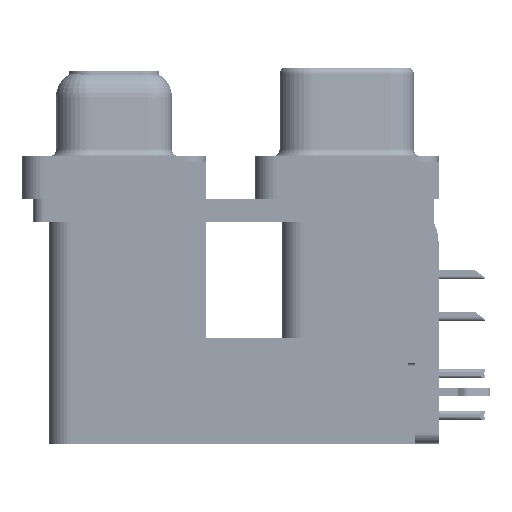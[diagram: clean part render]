
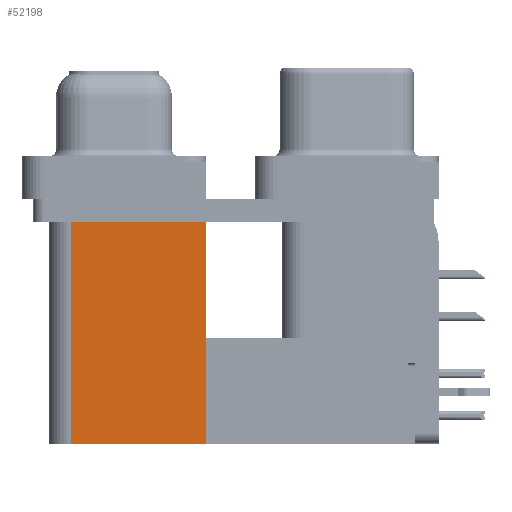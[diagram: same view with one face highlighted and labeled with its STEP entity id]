
A CAD part, left-side view. The second image highlights one B-rep face of the part: STEP entity #52198.
In plain terms, the highlighted planar face has unit normal (-1, 0, 0).
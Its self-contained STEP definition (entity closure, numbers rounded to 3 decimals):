
#2937 = CARTESIAN_POINT ( 'NONE',  ( 3.79, 18.8, -19.2 ) ) ;
#3347 = EDGE_LOOP ( 'NONE', ( #26915, #19031, #13800, #28448 ) ) ;
#3531 = EDGE_CURVE ( 'NONE', #57942, #61776, #18098, .T. ) ;
#4173 = CARTESIAN_POINT ( 'NONE',  ( 3.79, 9.6, -19.2 ) ) ;
#6087 = AXIS2_PLACEMENT_3D ( 'NONE', #23363, #63778, #54277 ) ;
#10407 = EDGE_CURVE ( 'NONE', #13706, #61776, #45657, .T. ) ;
#13706 = VERTEX_POINT ( 'NONE', #2937 ) ;
#13800 = ORIENTED_EDGE ( 'NONE', *, *, #35680, .F. ) ;
#14604 = CARTESIAN_POINT ( 'NONE',  ( 3.79, 18.8, -2.5 ) ) ;
#18098 = LINE ( 'NONE', #38801, #58396 ) ;
#19031 = ORIENTED_EDGE ( 'NONE', *, *, #10407, .F. ) ;
#21102 = CARTESIAN_POINT ( 'NONE',  ( 3.79, 9.6, -19.2 ) ) ;
#23363 = CARTESIAN_POINT ( 'NONE',  ( 3.79, 9.6, -19.2 ) ) ;
#26915 = ORIENTED_EDGE ( 'NONE', *, *, #3531, .T. ) ;
#27692 = EDGE_CURVE ( 'NONE', #57600, #57942, #54290, .T. ) ;
#28448 = ORIENTED_EDGE ( 'NONE', *, *, #27692, .T. ) ;
#29722 = CARTESIAN_POINT ( 'NONE',  ( 3.79, 18.8, -19.2 ) ) ;
#32843 = VECTOR ( 'NONE', #50386, 1000. ) ;
#35680 = EDGE_CURVE ( 'NONE', #57600, #13706, #51727, .T. ) ;
#38801 = CARTESIAN_POINT ( 'NONE',  ( 3.79, 9.6, -2.5 ) ) ;
#39457 = VECTOR ( 'NONE', #44085, 1000. ) ;
#43736 = PLANE ( 'NONE',  #6087 ) ;
#44085 = DIRECTION ( 'NONE',  ( 0., 0., 1. ) ) ;
#45657 = LINE ( 'NONE', #29722, #58118 ) ;
#49173 = CARTESIAN_POINT ( 'NONE',  ( 3.79, 9.6, -19.2 ) ) ;
#50386 = DIRECTION ( 'NONE',  ( 0., 1., 0. ) ) ;
#50420 = DIRECTION ( 'NONE',  ( 0., 0., 1. ) ) ;
#50895 = CARTESIAN_POINT ( 'NONE',  ( 3.79, 9.6, -2.5 ) ) ;
#51727 = LINE ( 'NONE', #4173, #32843 ) ;
#52198 = ADVANCED_FACE ( 'NONE', ( #53944 ), #43736, .F. ) ;
#53944 = FACE_OUTER_BOUND ( 'NONE', #3347, .T. ) ;
#54277 = DIRECTION ( 'NONE',  ( 0., 1., 0. ) ) ;
#54290 = LINE ( 'NONE', #49173, #39457 ) ;
#57600 = VERTEX_POINT ( 'NONE', #21102 ) ;
#57942 = VERTEX_POINT ( 'NONE', #50895 ) ;
#58118 = VECTOR ( 'NONE', #50420, 1000. ) ;
#58396 = VECTOR ( 'NONE', #59534, 1000. ) ;
#59534 = DIRECTION ( 'NONE',  ( 0., 1., 0. ) ) ;
#61776 = VERTEX_POINT ( 'NONE', #14604 ) ;
#63778 = DIRECTION ( 'NONE',  ( 1., 0., 0. ) ) ;
